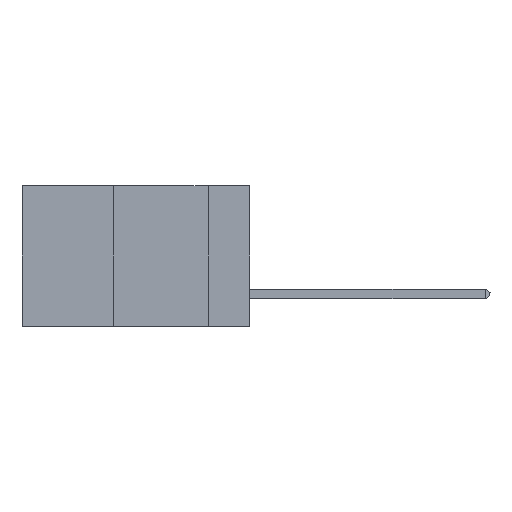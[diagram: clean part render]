
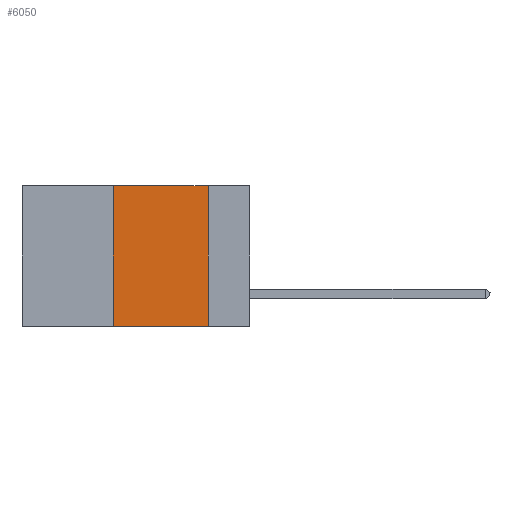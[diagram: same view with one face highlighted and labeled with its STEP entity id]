
A CAD part, left-side view. The second image highlights one B-rep face of the part: STEP entity #6050.
In plain terms, the highlighted planar face has unit normal (-1, 0, 0).
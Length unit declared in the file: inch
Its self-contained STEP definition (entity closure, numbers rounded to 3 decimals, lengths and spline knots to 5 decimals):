
#183 = VERTEX_POINT ( 'NONE', #18544 ) ;
#702 = AXIS2_PLACEMENT_3D ( 'NONE', #3790, #9667, #23497 ) ;
#1129 = CARTESIAN_POINT ( 'NONE',  ( 0., 0.36, 0. ) ) ;
#1723 = PLANE ( 'NONE',  #702 ) ;
#2210 = VERTEX_POINT ( 'NONE', #17601 ) ;
#2588 = DIRECTION ( 'NONE',  ( 0., -1., 0. ) ) ;
#2850 = DIRECTION ( 'NONE',  ( 0., 0., -1. ) ) ;
#3056 = ORIENTED_EDGE ( 'NONE', *, *, #20057, .F. ) ;
#3790 = CARTESIAN_POINT ( 'NONE',  ( 0., 0.6, 0. ) ) ;
#4283 = CARTESIAN_POINT ( 'NONE',  ( 0., 0.6, 0. ) ) ;
#4912 = VERTEX_POINT ( 'NONE', #25101 ) ;
#6050 = ADVANCED_FACE ( 'NONE', ( #18448 ), #1723, .F. ) ;
#6547 = EDGE_LOOP ( 'NONE', ( #22903, #3056, #20236, #25131 ) ) ;
#9374 = EDGE_CURVE ( 'NONE', #2210, #4912, #17472, .T. ) ;
#9667 = DIRECTION ( 'NONE',  ( 1., 0., 0. ) ) ;
#10559 = CARTESIAN_POINT ( 'NONE',  ( 0., 0.11, 0. ) ) ;
#10654 = VECTOR ( 'NONE', #12636, 39.37008 ) ;
#12636 = DIRECTION ( 'NONE',  ( 0., 0., 1. ) ) ;
#13549 = VECTOR ( 'NONE', #2588, 39.37008 ) ;
#14123 = LINE ( 'NONE', #16435, #13549 ) ;
#14444 = DIRECTION ( 'NONE',  ( 0., -1., 0. ) ) ;
#16338 = LINE ( 'NONE', #4283, #19119 ) ;
#16435 = CARTESIAN_POINT ( 'NONE',  ( 0., 0.6, -0.37 ) ) ;
#17472 = LINE ( 'NONE', #1129, #10654 ) ;
#17601 = CARTESIAN_POINT ( 'NONE',  ( 0., 0.36, -0.37 ) ) ;
#18448 = FACE_OUTER_BOUND ( 'NONE', #6547, .T. ) ;
#18544 = CARTESIAN_POINT ( 'NONE',  ( 0., 0.11, -0.37 ) ) ;
#19114 = EDGE_CURVE ( 'NONE', #20702, #183, #24722, .T. ) ;
#19119 = VECTOR ( 'NONE', #14444, 39.37008 ) ;
#20057 = EDGE_CURVE ( 'NONE', #4912, #20702, #16338, .T. ) ;
#20236 = ORIENTED_EDGE ( 'NONE', *, *, #9374, .F. ) ;
#20412 = VECTOR ( 'NONE', #2850, 39.37008 ) ;
#20702 = VERTEX_POINT ( 'NONE', #10559 ) ;
#20705 = EDGE_CURVE ( 'NONE', #2210, #183, #14123, .T. ) ;
#22903 = ORIENTED_EDGE ( 'NONE', *, *, #19114, .F. ) ;
#23497 = DIRECTION ( 'NONE',  ( 0., 0., -1. ) ) ;
#24376 = CARTESIAN_POINT ( 'NONE',  ( 0., 0.11, 0. ) ) ;
#24722 = LINE ( 'NONE', #24376, #20412 ) ;
#25101 = CARTESIAN_POINT ( 'NONE',  ( 0., 0.36, 0. ) ) ;
#25131 = ORIENTED_EDGE ( 'NONE', *, *, #20705, .T. ) ;
